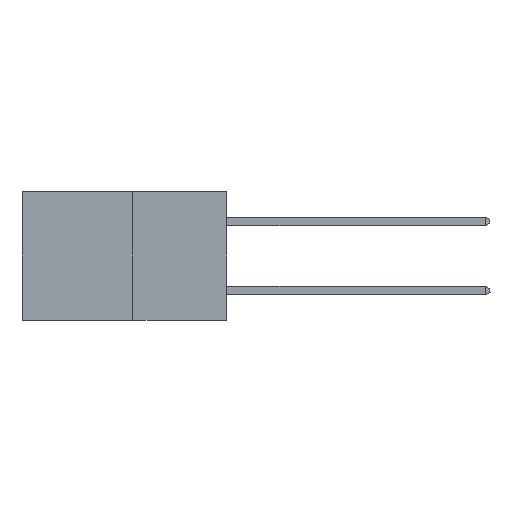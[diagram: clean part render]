
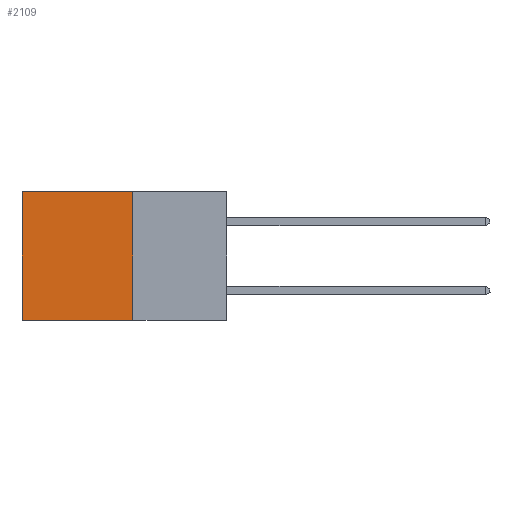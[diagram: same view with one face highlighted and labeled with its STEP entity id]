
A CAD part, left-side view. The second image highlights one B-rep face of the part: STEP entity #2109.
In plain terms, the highlighted planar face has unit normal (-1, 0, 0).
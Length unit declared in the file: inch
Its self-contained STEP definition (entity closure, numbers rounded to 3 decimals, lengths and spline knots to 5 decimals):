
#35 = CARTESIAN_POINT ( 'NONE',  ( 0.277, 0.27, -0.37 ) ) ;
#147 = VECTOR ( 'NONE', #9467, 39.37008 ) ;
#167 = DIRECTION ( 'NONE',  ( 0., 1., 0. ) ) ;
#287 = ORIENTED_EDGE ( 'NONE', *, *, #6522, .T. ) ;
#511 = VERTEX_POINT ( 'NONE', #6494 ) ;
#1312 = ORIENTED_EDGE ( 'NONE', *, *, #7393, .T. ) ;
#1781 = LINE ( 'NONE', #9266, #9282 ) ;
#1870 = VERTEX_POINT ( 'NONE', #6676 ) ;
#2007 = LINE ( 'NONE', #4023, #9416 ) ;
#2035 = AXIS2_PLACEMENT_3D ( 'NONE', #3488, #3486, #7893 ) ;
#2109 = ADVANCED_FACE ( 'NONE', ( #8385 ), #5420, .F. ) ;
#2230 = DIRECTION ( 'NONE',  ( 0., 0., -1. ) ) ;
#2480 = CARTESIAN_POINT ( 'NONE',  ( 0.277, 0.27, -0.37 ) ) ;
#2870 = CARTESIAN_POINT ( 'NONE',  ( 0.277, 0.59, -0.37 ) ) ;
#3086 = EDGE_CURVE ( 'NONE', #6973, #5253, #1781, .T. ) ;
#3183 = EDGE_LOOP ( 'NONE', ( #1312, #3274, #5809, #287 ) ) ;
#3274 = ORIENTED_EDGE ( 'NONE', *, *, #3086, .F. ) ;
#3486 = DIRECTION ( 'NONE',  ( 1., 0., 0. ) ) ;
#3488 = CARTESIAN_POINT ( 'NONE',  ( 0.277, 0.27, -0.37 ) ) ;
#3976 = DIRECTION ( 'NONE',  ( 0., 1., 0. ) ) ;
#4023 = CARTESIAN_POINT ( 'NONE',  ( 0.277, 0.27, 0. ) ) ;
#4790 = LINE ( 'NONE', #9166, #147 ) ;
#5253 = VERTEX_POINT ( 'NONE', #2870 ) ;
#5420 = PLANE ( 'NONE',  #2035 ) ;
#5500 = EDGE_CURVE ( 'NONE', #1870, #6973, #6656, .T. ) ;
#5809 = ORIENTED_EDGE ( 'NONE', *, *, #5500, .F. ) ;
#6494 = CARTESIAN_POINT ( 'NONE',  ( 0.277, 0.59, 0. ) ) ;
#6522 = EDGE_CURVE ( 'NONE', #1870, #511, #2007, .T. ) ;
#6656 = LINE ( 'NONE', #2480, #8361 ) ;
#6676 = CARTESIAN_POINT ( 'NONE',  ( 0.277, 0.27, 0. ) ) ;
#6973 = VERTEX_POINT ( 'NONE', #35 ) ;
#7393 = EDGE_CURVE ( 'NONE', #511, #5253, #4790, .T. ) ;
#7893 = DIRECTION ( 'NONE',  ( 0., 0., -1. ) ) ;
#8361 = VECTOR ( 'NONE', #2230, 39.37008 ) ;
#8385 = FACE_OUTER_BOUND ( 'NONE', #3183, .T. ) ;
#9166 = CARTESIAN_POINT ( 'NONE',  ( 0.277, 0.59, -0.37 ) ) ;
#9266 = CARTESIAN_POINT ( 'NONE',  ( 0.277, 0.27, -0.37 ) ) ;
#9282 = VECTOR ( 'NONE', #167, 39.37008 ) ;
#9416 = VECTOR ( 'NONE', #3976, 39.37008 ) ;
#9467 = DIRECTION ( 'NONE',  ( 0., 0., -1. ) ) ;
